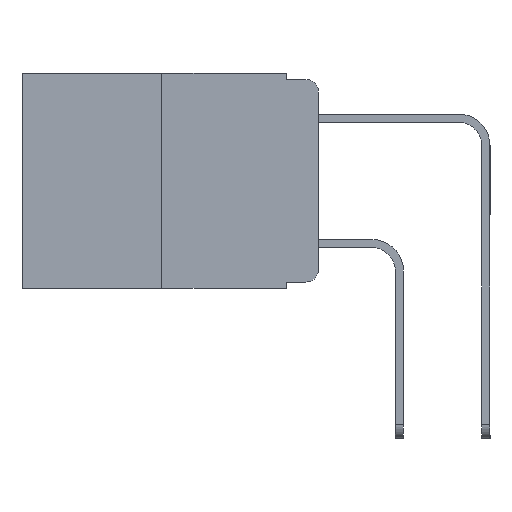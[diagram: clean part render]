
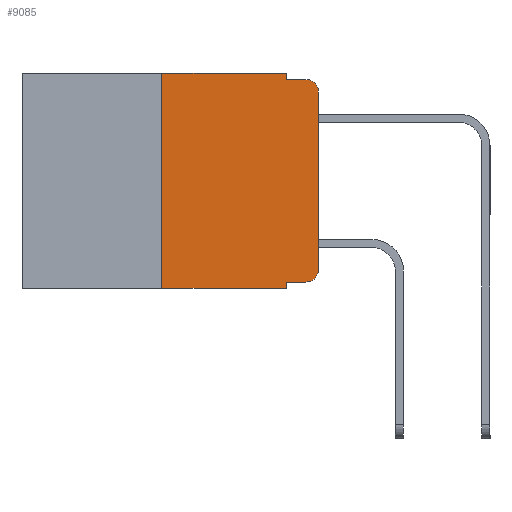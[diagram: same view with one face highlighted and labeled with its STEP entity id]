
A CAD part, left-side view. The second image highlights one B-rep face of the part: STEP entity #9085.
In plain terms, the highlighted planar face has unit normal (-1, 0, 0).
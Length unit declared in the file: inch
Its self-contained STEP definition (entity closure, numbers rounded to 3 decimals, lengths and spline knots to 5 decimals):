
#128 = VECTOR ( 'NONE', #3978, 39.37008 ) ;
#169 = DIRECTION ( 'NONE',  ( 1., 0., 0. ) ) ;
#276 = EDGE_CURVE ( 'NONE', #12023, #11801, #14523, .T. ) ;
#614 = EDGE_CURVE ( 'NONE', #3283, #9342, #15049, .T. ) ;
#818 = LINE ( 'NONE', #13245, #8121 ) ;
#888 = EDGE_CURVE ( 'NONE', #4805, #13580, #818, .T. ) ;
#949 = EDGE_LOOP ( 'NONE', ( #5107, #8792, #12615, #16057, #2107, #6433, #10009, #13828, #10806, #4455 ) ) ;
#1510 = CARTESIAN_POINT ( 'NONE',  ( 0., 0.051, 0. ) ) ;
#2107 = ORIENTED_EDGE ( 'NONE', *, *, #17099, .F. ) ;
#2200 = VECTOR ( 'NONE', #10623, 39.37008 ) ;
#2585 = CARTESIAN_POINT ( 'NONE',  ( 0., 0., -0.03 ) ) ;
#3283 = VERTEX_POINT ( 'NONE', #9275 ) ;
#3549 = CARTESIAN_POINT ( 'NONE',  ( 0., 0.02, -0.313 ) ) ;
#3599 = LINE ( 'NONE', #4989, #6877 ) ;
#3731 = EDGE_CURVE ( 'NONE', #11934, #17266, #15916, .T. ) ;
#3953 = CARTESIAN_POINT ( 'NONE',  ( 0., 0.051, -0.01 ) ) ;
#3978 = DIRECTION ( 'NONE',  ( 0., -1., 0. ) ) ;
#4122 = EDGE_CURVE ( 'NONE', #6065, #11801, #17532, .T. ) ;
#4455 = ORIENTED_EDGE ( 'NONE', *, *, #614, .T. ) ;
#4700 = LINE ( 'NONE', #6896, #12248 ) ;
#4805 = VERTEX_POINT ( 'NONE', #14414 ) ;
#4989 = CARTESIAN_POINT ( 'NONE',  ( 0., 0.473, -0.343 ) ) ;
#5107 = ORIENTED_EDGE ( 'NONE', *, *, #16199, .T. ) ;
#5910 = CARTESIAN_POINT ( 'NONE',  ( 0., 0.25, 0. ) ) ;
#6065 = VERTEX_POINT ( 'NONE', #10203 ) ;
#6316 = EDGE_CURVE ( 'NONE', #11934, #3283, #13109, .T. ) ;
#6433 = ORIENTED_EDGE ( 'NONE', *, *, #888, .F. ) ;
#6581 = DIRECTION ( 'NONE',  ( 0., 0., -1. ) ) ;
#6734 = CARTESIAN_POINT ( 'NONE',  ( 0., 0.051, -0.333 ) ) ;
#6773 = VERTEX_POINT ( 'NONE', #10063 ) ;
#6877 = VECTOR ( 'NONE', #12978, 39.37008 ) ;
#6896 = CARTESIAN_POINT ( 'NONE',  ( 0., 0.051, 0. ) ) ;
#7371 = AXIS2_PLACEMENT_3D ( 'NONE', #3549, #9305, #8744 ) ;
#7978 = CARTESIAN_POINT ( 'NONE',  ( 0., 0.051, -0.333 ) ) ;
#8121 = VECTOR ( 'NONE', #16519, 39.37008 ) ;
#8529 = CARTESIAN_POINT ( 'NONE',  ( 0., 0.051, -0.343 ) ) ;
#8744 = DIRECTION ( 'NONE',  ( 0., 0., -1. ) ) ;
#8792 = ORIENTED_EDGE ( 'NONE', *, *, #276, .T. ) ;
#8930 = CARTESIAN_POINT ( 'NONE',  ( 0., 0.473, 0. ) ) ;
#9085 = ADVANCED_FACE ( 'NONE', ( #15474 ), #16669, .F. ) ;
#9171 = LINE ( 'NONE', #16103, #15627 ) ;
#9208 = EDGE_CURVE ( 'NONE', #4805, #17266, #3599, .T. ) ;
#9275 = CARTESIAN_POINT ( 'NONE',  ( 0., 0.02, -0.333 ) ) ;
#9305 = DIRECTION ( 'NONE',  ( -1., 0., 0. ) ) ;
#9342 = VERTEX_POINT ( 'NONE', #17109 ) ;
#9361 = DIRECTION ( 'NONE',  ( 0., 0., 1. ) ) ;
#10009 = ORIENTED_EDGE ( 'NONE', *, *, #9208, .T. ) ;
#10063 = CARTESIAN_POINT ( 'NONE',  ( 0., 0.051, 0. ) ) ;
#10203 = CARTESIAN_POINT ( 'NONE',  ( 0., 0.051, -0.01 ) ) ;
#10236 = DIRECTION ( 'NONE',  ( 0., 0., -1. ) ) ;
#10623 = DIRECTION ( 'NONE',  ( 0., -1., 0. ) ) ;
#10806 = ORIENTED_EDGE ( 'NONE', *, *, #6316, .T. ) ;
#11768 = CARTESIAN_POINT ( 'NONE',  ( 0., 0.02, -0.01 ) ) ;
#11801 = VERTEX_POINT ( 'NONE', #11768 ) ;
#11934 = VERTEX_POINT ( 'NONE', #6734 ) ;
#12023 = VERTEX_POINT ( 'NONE', #2585 ) ;
#12248 = VECTOR ( 'NONE', #16045, 39.37008 ) ;
#12615 = ORIENTED_EDGE ( 'NONE', *, *, #4122, .F. ) ;
#12978 = DIRECTION ( 'NONE',  ( 0., -1., 0. ) ) ;
#13109 = LINE ( 'NONE', #7978, #2200 ) ;
#13225 = VECTOR ( 'NONE', #9361, 39.37008 ) ;
#13245 = CARTESIAN_POINT ( 'NONE',  ( 0., 0.25, 0. ) ) ;
#13580 = VERTEX_POINT ( 'NONE', #5910 ) ;
#13828 = ORIENTED_EDGE ( 'NONE', *, *, #3731, .F. ) ;
#14414 = CARTESIAN_POINT ( 'NONE',  ( 0., 0.25, -0.343 ) ) ;
#14523 = CIRCLE ( 'NONE', #15010, 0.02 ) ;
#14554 = AXIS2_PLACEMENT_3D ( 'NONE', #8930, #169, #10236 ) ;
#14803 = DIRECTION ( 'NONE',  ( 0., -1., 0. ) ) ;
#15007 = EDGE_CURVE ( 'NONE', #6773, #6065, #4700, .T. ) ;
#15010 = AXIS2_PLACEMENT_3D ( 'NONE', #17237, #17582, #6581 ) ;
#15049 = CIRCLE ( 'NONE', #7371, 0.02 ) ;
#15474 = FACE_OUTER_BOUND ( 'NONE', #949, .T. ) ;
#15503 = VECTOR ( 'NONE', #16493, 39.37008 ) ;
#15627 = VECTOR ( 'NONE', #14803, 39.37008 ) ;
#15916 = LINE ( 'NONE', #1510, #15503 ) ;
#16045 = DIRECTION ( 'NONE',  ( 0., 0., -1. ) ) ;
#16057 = ORIENTED_EDGE ( 'NONE', *, *, #15007, .F. ) ;
#16103 = CARTESIAN_POINT ( 'NONE',  ( 0., 0.473, 0. ) ) ;
#16199 = EDGE_CURVE ( 'NONE', #9342, #12023, #16264, .T. ) ;
#16264 = LINE ( 'NONE', #17105, #13225 ) ;
#16493 = DIRECTION ( 'NONE',  ( 0., 0., -1. ) ) ;
#16519 = DIRECTION ( 'NONE',  ( 0., 0., 1. ) ) ;
#16669 = PLANE ( 'NONE',  #14554 ) ;
#17099 = EDGE_CURVE ( 'NONE', #13580, #6773, #9171, .T. ) ;
#17105 = CARTESIAN_POINT ( 'NONE',  ( 0., 0., 0. ) ) ;
#17109 = CARTESIAN_POINT ( 'NONE',  ( 0., 0., -0.313 ) ) ;
#17237 = CARTESIAN_POINT ( 'NONE',  ( 0., 0.02, -0.03 ) ) ;
#17266 = VERTEX_POINT ( 'NONE', #8529 ) ;
#17532 = LINE ( 'NONE', #3953, #128 ) ;
#17582 = DIRECTION ( 'NONE',  ( -1., 0., 0. ) ) ;
